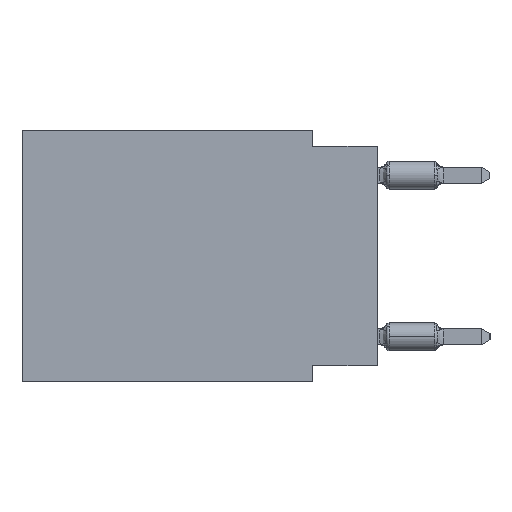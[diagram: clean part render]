
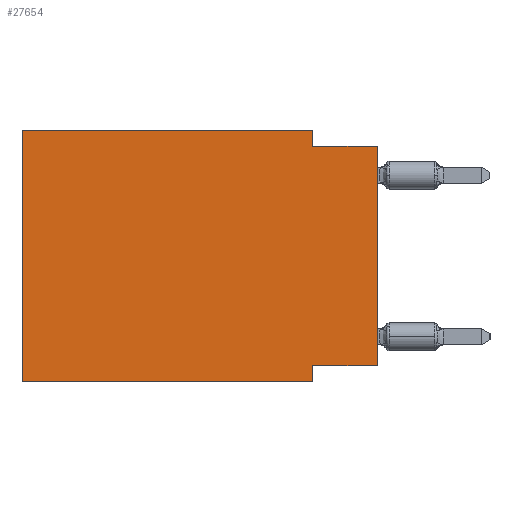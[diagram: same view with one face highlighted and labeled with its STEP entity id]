
A CAD part, left-side view. The second image highlights one B-rep face of the part: STEP entity #27654.
In plain terms, the highlighted planar face has unit normal (-1, 0, 0).
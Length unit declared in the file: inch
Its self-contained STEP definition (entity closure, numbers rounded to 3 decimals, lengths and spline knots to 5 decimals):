
#577 = DIRECTION ( 'NONE',  ( 1., 0., 0. ) ) ;
#658 = EDGE_CURVE ( 'NONE', #8622, #25141, #32213, .T. ) ;
#717 = VECTOR ( 'NONE', #19468, 39.37008 ) ;
#2499 = EDGE_CURVE ( 'NONE', #18613, #17168, #20989, .T. ) ;
#2522 = LINE ( 'NONE', #49548, #717 ) ;
#2671 = CARTESIAN_POINT ( 'NONE',  ( 0., 0.1, -0.39 ) ) ;
#3015 = CARTESIAN_POINT ( 'NONE',  ( 0., 0.1, 0. ) ) ;
#3528 = VECTOR ( 'NONE', #44966, 39.37008 ) ;
#5261 = CARTESIAN_POINT ( 'NONE',  ( 0., 0.55, 0. ) ) ;
#5348 = LINE ( 'NONE', #18118, #39367 ) ;
#6347 = VERTEX_POINT ( 'NONE', #51106 ) ;
#6351 = CARTESIAN_POINT ( 'NONE',  ( 0., 0., -0.365 ) ) ;
#7342 = ORIENTED_EDGE ( 'NONE', *, *, #23553, .F. ) ;
#7370 = CARTESIAN_POINT ( 'NONE',  ( 0., 0., -0.025 ) ) ;
#7834 = ORIENTED_EDGE ( 'NONE', *, *, #2499, .F. ) ;
#8622 = VERTEX_POINT ( 'NONE', #19212 ) ;
#8946 = PLANE ( 'NONE',  #35802 ) ;
#15253 = CARTESIAN_POINT ( 'NONE',  ( 0., 0.1, -0.39 ) ) ;
#16126 = LINE ( 'NONE', #24728, #41984 ) ;
#16870 = CARTESIAN_POINT ( 'NONE',  ( 0., 0.1, -0.025 ) ) ;
#17168 = VERTEX_POINT ( 'NONE', #5261 ) ;
#18118 = CARTESIAN_POINT ( 'NONE',  ( 0., 0.1, 0. ) ) ;
#18613 = VERTEX_POINT ( 'NONE', #29697 ) ;
#19212 = CARTESIAN_POINT ( 'NONE',  ( 0., 0., -0.365 ) ) ;
#19468 = DIRECTION ( 'NONE',  ( 0., 0., 1. ) ) ;
#20401 = VERTEX_POINT ( 'NONE', #16870 ) ;
#20806 = DIRECTION ( 'NONE',  ( 0., 0., -1. ) ) ;
#20989 = LINE ( 'NONE', #25441, #24497 ) ;
#21706 = CARTESIAN_POINT ( 'NONE',  ( 0., 0.55, 0. ) ) ;
#23553 = EDGE_CURVE ( 'NONE', #20401, #6347, #36869, .T. ) ;
#23837 = DIRECTION ( 'NONE',  ( 0., 1., 0. ) ) ;
#24497 = VECTOR ( 'NONE', #37717, 39.37008 ) ;
#24728 = CARTESIAN_POINT ( 'NONE',  ( 0., 0.55, 0. ) ) ;
#25141 = VERTEX_POINT ( 'NONE', #30427 ) ;
#25441 = CARTESIAN_POINT ( 'NONE',  ( 0., 0.55, 0. ) ) ;
#26857 = EDGE_CURVE ( 'NONE', #17168, #40587, #16126, .T. ) ;
#27654 = ADVANCED_FACE ( 'NONE', ( #34800 ), #8946, .F. ) ;
#29697 = CARTESIAN_POINT ( 'NONE',  ( 0., 0.55, -0.39 ) ) ;
#29891 = CARTESIAN_POINT ( 'NONE',  ( 0., 0.55, -0.39 ) ) ;
#30344 = DIRECTION ( 'NONE',  ( 0., 0., -1. ) ) ;
#30427 = CARTESIAN_POINT ( 'NONE',  ( 0., 0.1, -0.365 ) ) ;
#32046 = EDGE_CURVE ( 'NONE', #8622, #6347, #2522, .T. ) ;
#32213 = LINE ( 'NONE', #6351, #36710 ) ;
#33118 = DIRECTION ( 'NONE',  ( 0., -1., 0. ) ) ;
#34800 = FACE_OUTER_BOUND ( 'NONE', #35190, .T. ) ;
#35107 = DIRECTION ( 'NONE',  ( 0., 0., -1. ) ) ;
#35190 = EDGE_LOOP ( 'NONE', ( #52139, #7342, #38876, #39030, #7834, #42056, #45096, #49485 ) ) ;
#35802 = AXIS2_PLACEMENT_3D ( 'NONE', #21706, #577, #30344 ) ;
#36710 = VECTOR ( 'NONE', #23837, 39.37008 ) ;
#36869 = LINE ( 'NONE', #7370, #3528 ) ;
#37057 = VECTOR ( 'NONE', #39617, 39.37008 ) ;
#37717 = DIRECTION ( 'NONE',  ( 0., 0., 1. ) ) ;
#38876 = ORIENTED_EDGE ( 'NONE', *, *, #40111, .F. ) ;
#39030 = ORIENTED_EDGE ( 'NONE', *, *, #26857, .F. ) ;
#39367 = VECTOR ( 'NONE', #35107, 39.37008 ) ;
#39617 = DIRECTION ( 'NONE',  ( 0., -1., 0. ) ) ;
#40111 = EDGE_CURVE ( 'NONE', #40587, #20401, #5348, .T. ) ;
#40587 = VERTEX_POINT ( 'NONE', #3015 ) ;
#41892 = EDGE_CURVE ( 'NONE', #25141, #50074, #53409, .T. ) ;
#41984 = VECTOR ( 'NONE', #33118, 39.37008 ) ;
#42056 = ORIENTED_EDGE ( 'NONE', *, *, #51452, .T. ) ;
#43001 = LINE ( 'NONE', #29891, #37057 ) ;
#44966 = DIRECTION ( 'NONE',  ( 0., -1., 0. ) ) ;
#45096 = ORIENTED_EDGE ( 'NONE', *, *, #41892, .F. ) ;
#46487 = VECTOR ( 'NONE', #20806, 39.37008 ) ;
#49485 = ORIENTED_EDGE ( 'NONE', *, *, #658, .F. ) ;
#49548 = CARTESIAN_POINT ( 'NONE',  ( 0., 0., 0. ) ) ;
#50074 = VERTEX_POINT ( 'NONE', #2671 ) ;
#51106 = CARTESIAN_POINT ( 'NONE',  ( 0., 0., -0.025 ) ) ;
#51452 = EDGE_CURVE ( 'NONE', #18613, #50074, #43001, .T. ) ;
#52139 = ORIENTED_EDGE ( 'NONE', *, *, #32046, .T. ) ;
#53409 = LINE ( 'NONE', #15253, #46487 ) ;
